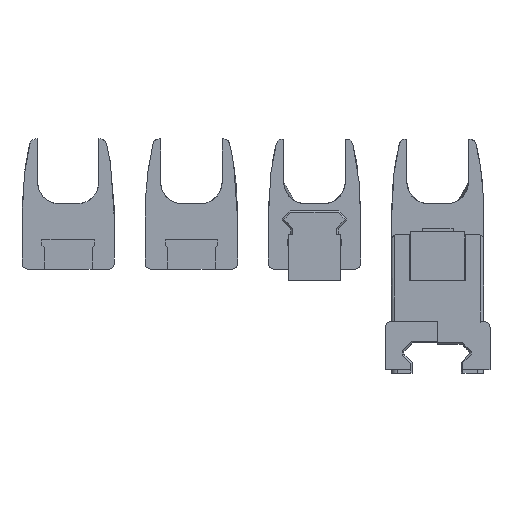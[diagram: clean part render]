
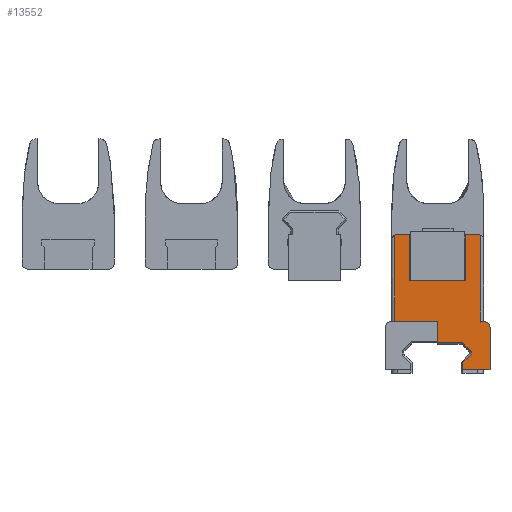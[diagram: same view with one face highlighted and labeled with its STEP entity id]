
A CAD part, front view. The second image highlights one B-rep face of the part: STEP entity #13552.
In plain terms, the highlighted planar face has unit normal (0, -1, 0).
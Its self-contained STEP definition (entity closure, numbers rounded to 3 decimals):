
#657=CIRCLE('',#14444,2.);
#658=CIRCLE('',#14447,2.);
#659=CIRCLE('',#14448,2.);
#1277=FACE_OUTER_BOUND('',#2047,.T.);
#2047=EDGE_LOOP('',(#11671,#11672,#11673,#11674,#11675,#11676,#11677,#11678,
#11679,#11680,#11681,#11682,#11683,#11684,#11685,#11686,#11687,#11688,#11689));
#3479=LINE('',#24663,#5003);
#3481=LINE('',#24678,#5005);
#3482=LINE('',#24680,#5006);
#3483=LINE('',#24682,#5007);
#3484=LINE('',#24684,#5008);
#3485=LINE('',#24686,#5009);
#3486=LINE('',#24690,#5010);
#3487=LINE('',#24692,#5011);
#3488=LINE('',#24694,#5012);
#3489=LINE('',#24696,#5013);
#3490=LINE('',#24698,#5014);
#3491=LINE('',#24700,#5015);
#3492=LINE('',#24702,#5016);
#3493=LINE('',#24704,#5017);
#3494=LINE('',#24706,#5018);
#3495=LINE('',#24708,#5019);
#5003=VECTOR('',#17412,10.);
#5005=VECTOR('',#17416,10.);
#5006=VECTOR('',#17417,10.);
#5007=VECTOR('',#17418,10.);
#5008=VECTOR('',#17419,10.);
#5009=VECTOR('',#17420,10.);
#5010=VECTOR('',#17423,10.);
#5011=VECTOR('',#17424,10.);
#5012=VECTOR('',#17425,10.);
#5013=VECTOR('',#17426,10.);
#5014=VECTOR('',#17427,10.);
#5015=VECTOR('',#17428,10.);
#5016=VECTOR('',#17429,10.);
#5017=VECTOR('',#17430,10.);
#5018=VECTOR('',#17431,10.);
#5019=VECTOR('',#17432,10.);
#6314=VERTEX_POINT('',#24642);
#6318=VERTEX_POINT('',#24658);
#6319=VERTEX_POINT('',#24662);
#6321=VERTEX_POINT('',#24677);
#6322=VERTEX_POINT('',#24679);
#6323=VERTEX_POINT('',#24681);
#6324=VERTEX_POINT('',#24683);
#6325=VERTEX_POINT('',#24685);
#6326=VERTEX_POINT('',#24687);
#6327=VERTEX_POINT('',#24689);
#6328=VERTEX_POINT('',#24691);
#6329=VERTEX_POINT('',#24693);
#6330=VERTEX_POINT('',#24695);
#6331=VERTEX_POINT('',#24697);
#6332=VERTEX_POINT('',#24699);
#6333=VERTEX_POINT('',#24701);
#6334=VERTEX_POINT('',#24703);
#6335=VERTEX_POINT('',#24705);
#6336=VERTEX_POINT('',#24707);
#8152=EDGE_CURVE('',#6318,#6314,#657,.T.);
#8153=EDGE_CURVE('',#6314,#6319,#3479,.T.);
#8156=EDGE_CURVE('',#6318,#6321,#3481,.T.);
#8157=EDGE_CURVE('',#6321,#6322,#3482,.T.);
#8158=EDGE_CURVE('',#6322,#6323,#3483,.T.);
#8159=EDGE_CURVE('',#6323,#6324,#3484,.T.);
#8160=EDGE_CURVE('',#6324,#6325,#3485,.T.);
#8161=EDGE_CURVE('',#6326,#6325,#658,.T.);
#8162=EDGE_CURVE('',#6327,#6326,#3486,.T.);
#8163=EDGE_CURVE('',#6327,#6328,#3487,.T.);
#8164=EDGE_CURVE('',#6328,#6329,#3488,.T.);
#8165=EDGE_CURVE('',#6330,#6329,#3489,.T.);
#8166=EDGE_CURVE('',#6331,#6330,#3490,.T.);
#8167=EDGE_CURVE('',#6332,#6331,#3491,.T.);
#8168=EDGE_CURVE('',#6333,#6332,#3492,.T.);
#8169=EDGE_CURVE('',#6334,#6333,#3493,.T.);
#8170=EDGE_CURVE('',#6334,#6335,#3494,.T.);
#8171=EDGE_CURVE('',#6335,#6336,#3495,.T.);
#8172=EDGE_CURVE('',#6319,#6336,#659,.T.);
#11671=ORIENTED_EDGE('',*,*,#8152,.F.);
#11672=ORIENTED_EDGE('',*,*,#8156,.T.);
#11673=ORIENTED_EDGE('',*,*,#8157,.T.);
#11674=ORIENTED_EDGE('',*,*,#8158,.T.);
#11675=ORIENTED_EDGE('',*,*,#8159,.T.);
#11676=ORIENTED_EDGE('',*,*,#8160,.T.);
#11677=ORIENTED_EDGE('',*,*,#8161,.F.);
#11678=ORIENTED_EDGE('',*,*,#8162,.F.);
#11679=ORIENTED_EDGE('',*,*,#8163,.T.);
#11680=ORIENTED_EDGE('',*,*,#8164,.T.);
#11681=ORIENTED_EDGE('',*,*,#8165,.F.);
#11682=ORIENTED_EDGE('',*,*,#8166,.F.);
#11683=ORIENTED_EDGE('',*,*,#8167,.F.);
#11684=ORIENTED_EDGE('',*,*,#8168,.F.);
#11685=ORIENTED_EDGE('',*,*,#8169,.F.);
#11686=ORIENTED_EDGE('',*,*,#8170,.T.);
#11687=ORIENTED_EDGE('',*,*,#8171,.T.);
#11688=ORIENTED_EDGE('',*,*,#8172,.F.);
#11689=ORIENTED_EDGE('',*,*,#8153,.F.);
#12884=PLANE('',#14446);
#13552=ADVANCED_FACE('',(#1277),#12884,.T.);
#14444=AXIS2_PLACEMENT_3D('',#24660,#17408,#17409);
#14446=AXIS2_PLACEMENT_3D('',#24676,#17414,#17415);
#14447=AXIS2_PLACEMENT_3D('',#24688,#17421,#17422);
#14448=AXIS2_PLACEMENT_3D('',#24709,#17433,#17434);
#17408=DIRECTION('center_axis',(0.,1.,0.));
#17409=DIRECTION('ref_axis',(0.707,0.,0.707));
#17412=DIRECTION('',(0.,0.,-1.));
#17414=DIRECTION('center_axis',(0.,-1.,0.));
#17415=DIRECTION('ref_axis',(0.,0.,-1.));
#17416=DIRECTION('',(-1.,0.,0.));
#17417=DIRECTION('',(0.,0.,-1.));
#17418=DIRECTION('',(-1.,0.,0.));
#17419=DIRECTION('',(0.,0.,1.));
#17420=DIRECTION('',(-1.,0.,0.));
#17421=DIRECTION('center_axis',(0.,1.,0.));
#17422=DIRECTION('ref_axis',(-0.707,0.,0.707));
#17423=DIRECTION('',(0.,0.,1.));
#17424=DIRECTION('',(1.,0.,0.));
#17425=DIRECTION('',(0.,0.,-1.));
#17426=DIRECTION('',(-1.,0.,0.));
#17427=DIRECTION('',(-0.707,0.,0.707));
#17428=DIRECTION('',(0.,0.,1.));
#17429=DIRECTION('',(0.707,0.,0.707));
#17430=DIRECTION('',(0.,0.,1.));
#17431=DIRECTION('',(1.,0.,0.));
#17432=DIRECTION('',(0.,0.,1.));
#17433=DIRECTION('center_axis',(0.,1.,0.));
#17434=DIRECTION('ref_axis',(0.707,0.,0.707));
#24642=CARTESIAN_POINT('',(229.,10.,14.732));
#24658=CARTESIAN_POINT('',(228.,10.,15.));
#24660=CARTESIAN_POINT('Origin',(228.,10.,13.));
#24662=CARTESIAN_POINT('',(229.,10.,-13.446));
#24663=CARTESIAN_POINT('',(229.,10.,-14.));
#24676=CARTESIAN_POINT('Origin',(230.,10.,-14.));
#24677=CARTESIAN_POINT('',(224.,10.,15.));
#24678=CARTESIAN_POINT('',(218.657,10.,15.));
#24679=CARTESIAN_POINT('',(224.,10.,0.));
#24680=CARTESIAN_POINT('',(224.,10.,0.5));
#24681=CARTESIAN_POINT('',(206.,10.,0.));
#24682=CARTESIAN_POINT('',(222.5,10.,0.));
#24683=CARTESIAN_POINT('',(206.,10.,15.));
#24684=CARTESIAN_POINT('',(206.,10.,0.5));
#24685=CARTESIAN_POINT('',(202.,10.,15.));
#24686=CARTESIAN_POINT('',(218.657,10.,15.));
#24687=CARTESIAN_POINT('',(201.,10.,14.732));
#24688=CARTESIAN_POINT('Origin',(202.,10.,13.));
#24689=CARTESIAN_POINT('',(201.,10.,-13.178));
#24690=CARTESIAN_POINT('',(201.,10.,4.5));
#24691=CARTESIAN_POINT('',(215.,10.,-13.178));
#24692=CARTESIAN_POINT('',(207.5,10.,-13.178));
#24693=CARTESIAN_POINT('',(215.,10.,-20.178));
#24694=CARTESIAN_POINT('',(215.,10.,7.411));
#24695=CARTESIAN_POINT('',(223.134,10.,-20.178));
#24696=CARTESIAN_POINT('',(203.536,10.,-20.178));
#24697=CARTESIAN_POINT('',(225.955,10.,-22.998));
#24698=CARTESIAN_POINT('',(204.879,10.,-1.923));
#24699=CARTESIAN_POINT('',(225.955,10.,-23.946));
#24700=CARTESIAN_POINT('',(225.955,10.,3.397));
#24701=CARTESIAN_POINT('',(223.186,10.,-26.715));
#24702=CARTESIAN_POINT('',(232.879,10.,-17.021));
#24703=CARTESIAN_POINT('',(223.186,10.,-29.));
#24704=CARTESIAN_POINT('',(223.186,10.,1.746));
#24705=CARTESIAN_POINT('',(232.,10.,-29.));
#24706=CARTESIAN_POINT('',(230.,10.,-29.));
#24707=CARTESIAN_POINT('',(232.,10.,-15.178));
#24708=CARTESIAN_POINT('',(232.,10.,-16.));
#24709=CARTESIAN_POINT('Origin',(230.,10.,-15.178));
